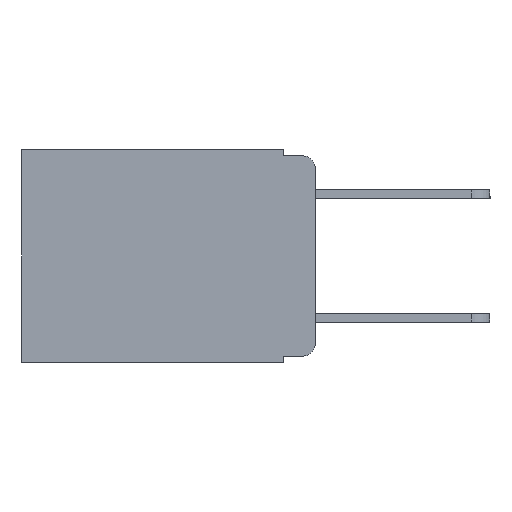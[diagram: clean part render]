
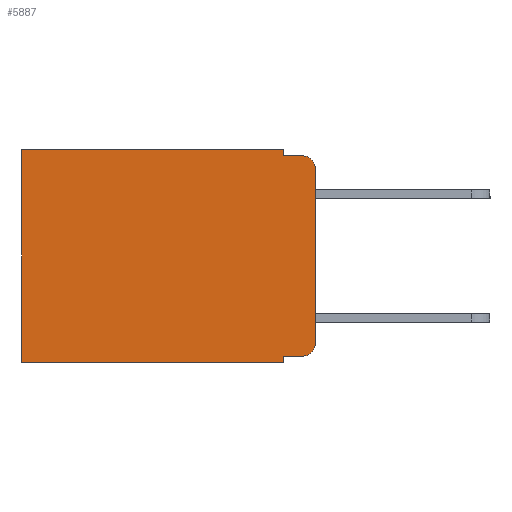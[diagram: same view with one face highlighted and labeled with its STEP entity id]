
A CAD part, left-side view. The second image highlights one B-rep face of the part: STEP entity #5887.
In plain terms, the highlighted planar face has unit normal (-1, 0, 0).
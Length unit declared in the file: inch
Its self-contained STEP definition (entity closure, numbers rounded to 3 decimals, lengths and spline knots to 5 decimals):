
#26 = AXIS2_PLACEMENT_3D ( 'NONE', #2787, #1467, #6550 ) ;
#74 = ORIENTED_EDGE ( 'NONE', *, *, #490, .T. ) ;
#129 = CARTESIAN_POINT ( 'NONE',  ( 0.298, 0.473, -0.343 ) ) ;
#255 = ORIENTED_EDGE ( 'NONE', *, *, #924, .T. ) ;
#373 = VERTEX_POINT ( 'NONE', #8782 ) ;
#384 = EDGE_CURVE ( 'NONE', #6157, #7504, #3316, .T. ) ;
#473 = EDGE_CURVE ( 'NONE', #5354, #10823, #10439, .T. ) ;
#490 = EDGE_CURVE ( 'NONE', #10561, #10823, #4915, .T. ) ;
#497 = EDGE_CURVE ( 'NONE', #10561, #3390, #9862, .T. ) ;
#773 = CARTESIAN_POINT ( 'NONE',  ( 0.298, 0., 0. ) ) ;
#790 = EDGE_CURVE ( 'NONE', #7643, #7504, #11562, .T. ) ;
#924 = EDGE_CURVE ( 'NONE', #373, #7643, #1510, .T. ) ;
#939 = CARTESIAN_POINT ( 'NONE',  ( 0.298, 0.051, -0.01 ) ) ;
#1260 = LINE ( 'NONE', #3480, #11188 ) ;
#1417 = EDGE_CURVE ( 'NONE', #373, #5354, #6962, .T. ) ;
#1467 = DIRECTION ( 'NONE',  ( -1., 0., 0. ) ) ;
#1468 = ORIENTED_EDGE ( 'NONE', *, *, #384, .F. ) ;
#1470 = CARTESIAN_POINT ( 'NONE',  ( 0.298, 0.02, -0.01 ) ) ;
#1510 = LINE ( 'NONE', #10885, #11690 ) ;
#1873 = VECTOR ( 'NONE', #1906, 39.37008 ) ;
#1882 = CARTESIAN_POINT ( 'NONE',  ( 0.298, 0.02, -0.333 ) ) ;
#1906 = DIRECTION ( 'NONE',  ( 0., 0., -1. ) ) ;
#2075 = VERTEX_POINT ( 'NONE', #9278 ) ;
#2422 = CARTESIAN_POINT ( 'NONE',  ( 0.298, 0.051, 0. ) ) ;
#2515 = CARTESIAN_POINT ( 'NONE',  ( 0.298, 0., -0.343 ) ) ;
#2517 = VECTOR ( 'NONE', #7893, 39.37008 ) ;
#2564 = DIRECTION ( 'NONE',  ( 0., 1., 0. ) ) ;
#2640 = EDGE_LOOP ( 'NONE', ( #2862, #74, #10414, #2893, #255, #3458, #1468, #3278, #2777, #4758 ) ) ;
#2777 = ORIENTED_EDGE ( 'NONE', *, *, #5923, .T. ) ;
#2787 = CARTESIAN_POINT ( 'NONE',  ( 0.298, 0.02, -0.03 ) ) ;
#2803 = DIRECTION ( 'NONE',  ( -1., 0., 0. ) ) ;
#2862 = ORIENTED_EDGE ( 'NONE', *, *, #497, .F. ) ;
#2885 = CARTESIAN_POINT ( 'NONE',  ( 0.298, 0.02, -0.313 ) ) ;
#2893 = ORIENTED_EDGE ( 'NONE', *, *, #1417, .F. ) ;
#3278 = ORIENTED_EDGE ( 'NONE', *, *, #4077, .F. ) ;
#3316 = LINE ( 'NONE', #2515, #10807 ) ;
#3390 = VERTEX_POINT ( 'NONE', #8302 ) ;
#3458 = ORIENTED_EDGE ( 'NONE', *, *, #790, .T. ) ;
#3480 = CARTESIAN_POINT ( 'NONE',  ( 0.298, 0.051, 0. ) ) ;
#3587 = EDGE_CURVE ( 'NONE', #5030, #3390, #10374, .T. ) ;
#4077 = EDGE_CURVE ( 'NONE', #2075, #6157, #1260, .T. ) ;
#4168 = CARTESIAN_POINT ( 'NONE',  ( 0.298, 0.051, -0.343 ) ) ;
#4724 = CARTESIAN_POINT ( 'NONE',  ( 0.298, 0.473, 0. ) ) ;
#4758 = ORIENTED_EDGE ( 'NONE', *, *, #3587, .T. ) ;
#4915 = CIRCLE ( 'NONE', #26, 0.02 ) ;
#5030 = VERTEX_POINT ( 'NONE', #1882 ) ;
#5339 = DIRECTION ( 'NONE',  ( 0., -1., 0. ) ) ;
#5354 = VERTEX_POINT ( 'NONE', #5889 ) ;
#5385 = PLANE ( 'NONE',  #11870 ) ;
#5388 = DIRECTION ( 'NONE',  ( 1., 0., 0. ) ) ;
#5441 = CARTESIAN_POINT ( 'NONE',  ( 0.298, 0.051, -0.333 ) ) ;
#5848 = CARTESIAN_POINT ( 'NONE',  ( 0.298, 0.473, 0. ) ) ;
#5887 = ADVANCED_FACE ( 'NONE', ( #8008 ), #5385, .F. ) ;
#5889 = CARTESIAN_POINT ( 'NONE',  ( 0.298, 0.051, -0.01 ) ) ;
#5923 = EDGE_CURVE ( 'NONE', #2075, #5030, #7700, .T. ) ;
#6157 = VERTEX_POINT ( 'NONE', #4168 ) ;
#6303 = DIRECTION ( 'NONE',  ( 0., 0., -1. ) ) ;
#6387 = CARTESIAN_POINT ( 'NONE',  ( 0.298, 0., 0. ) ) ;
#6550 = DIRECTION ( 'NONE',  ( 0., 0., -1. ) ) ;
#6946 = DIRECTION ( 'NONE',  ( 0., 1., 0. ) ) ;
#6962 = LINE ( 'NONE', #2422, #9210 ) ;
#7504 = VERTEX_POINT ( 'NONE', #129 ) ;
#7631 = DIRECTION ( 'NONE',  ( 0., 0., -1. ) ) ;
#7643 = VERTEX_POINT ( 'NONE', #5848 ) ;
#7700 = LINE ( 'NONE', #5441, #12059 ) ;
#7893 = DIRECTION ( 'NONE',  ( 0., -1., 0. ) ) ;
#8008 = FACE_OUTER_BOUND ( 'NONE', #2640, .T. ) ;
#8302 = CARTESIAN_POINT ( 'NONE',  ( 0.298, 0., -0.313 ) ) ;
#8773 = VECTOR ( 'NONE', #11361, 39.37008 ) ;
#8780 = DIRECTION ( 'NONE',  ( 0., 0., -1. ) ) ;
#8782 = CARTESIAN_POINT ( 'NONE',  ( 0.298, 0.051, 0. ) ) ;
#9210 = VECTOR ( 'NONE', #8780, 39.37008 ) ;
#9278 = CARTESIAN_POINT ( 'NONE',  ( 0.298, 0.051, -0.333 ) ) ;
#9472 = DIRECTION ( 'NONE',  ( 0., 0., -1. ) ) ;
#9862 = LINE ( 'NONE', #773, #1873 ) ;
#10374 = CIRCLE ( 'NONE', #11949, 0.02 ) ;
#10414 = ORIENTED_EDGE ( 'NONE', *, *, #473, .F. ) ;
#10439 = LINE ( 'NONE', #939, #2517 ) ;
#10561 = VERTEX_POINT ( 'NONE', #12833 ) ;
#10807 = VECTOR ( 'NONE', #2564, 39.37008 ) ;
#10823 = VERTEX_POINT ( 'NONE', #1470 ) ;
#10885 = CARTESIAN_POINT ( 'NONE',  ( 0.298, 0., 0. ) ) ;
#11188 = VECTOR ( 'NONE', #9472, 39.37008 ) ;
#11361 = DIRECTION ( 'NONE',  ( 0., 0., -1. ) ) ;
#11562 = LINE ( 'NONE', #4724, #8773 ) ;
#11690 = VECTOR ( 'NONE', #6946, 39.37008 ) ;
#11870 = AXIS2_PLACEMENT_3D ( 'NONE', #6387, #5388, #7631 ) ;
#11949 = AXIS2_PLACEMENT_3D ( 'NONE', #2885, #2803, #6303 ) ;
#12059 = VECTOR ( 'NONE', #5339, 39.37008 ) ;
#12833 = CARTESIAN_POINT ( 'NONE',  ( 0.298, 0., -0.03 ) ) ;
